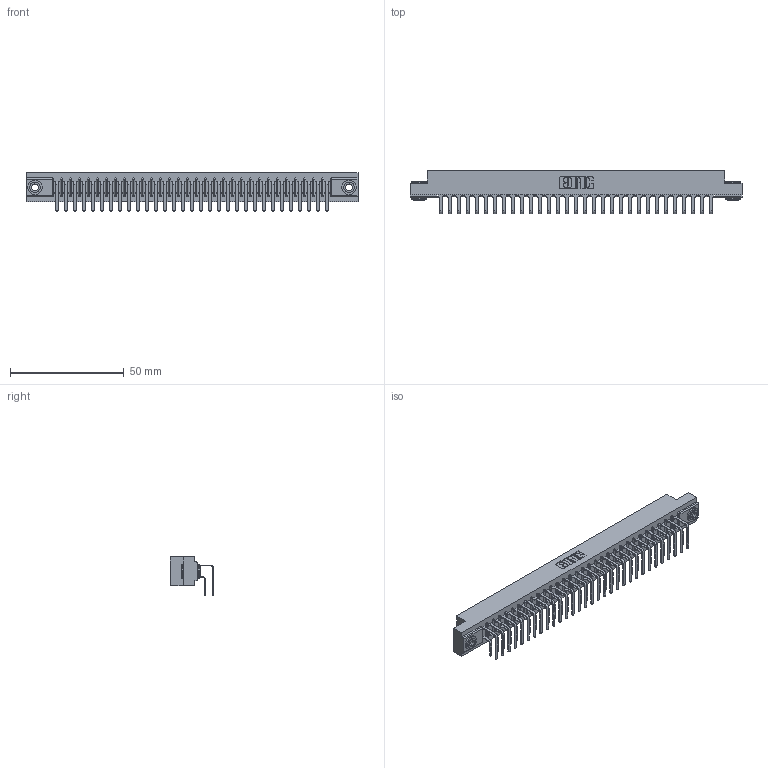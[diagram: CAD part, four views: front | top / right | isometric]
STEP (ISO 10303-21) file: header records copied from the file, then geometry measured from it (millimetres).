
FILE_DESCRIPTION (( 'STEP AP203' ), '1' );
FILE_NAME ('307-062-458-203.STEP', '2020-09-30T16:51:52', ( '' ), ( '' ), 'SwSTEP 2.0', 'SolidWorks 2020', '' );
FILE_SCHEMA (( 'CONFIG_CONTROL_DESIGN' ));
Length unit declared in the file: inch
Products named in the file (5): 307-062-458-203; 307-290-001_558 559 - 1 (Single); 345-250-002_345-250-002-102; 307 Part_.156 Dia Mounting Holes; 307-290-001_558 - 2 (Single)
Assembly tree (65 placements, depth 2):
  307-062-458-203
    307 Part_.156 Dia Mounting Holes
    307-290-001_558 559 - 1 (Single)  x31
    307-290-001_558 - 2 (Single)  x31
    345-250-002_345-250-002-102  x2
Bounding box: 145.85 x 18.96 x 16.8 mm (x, y, z)
Volume: 15707.3 mm3; surface area: 20848.5 mm2
Topology: 65 solids, 65 shells, 3302 faces, 9239 edges, 5986 vertices
Faces by surface type: plane 2140, cylinder 1090, sphere 64, cone 8
Entity records: 31436 total; most frequent: CARTESIAN_POINT 5130, ORIENTED_EDGE 5074, DIRECTION 5043, EDGE_CURVE 2537, VECTOR 1933, LINE 1933, VERTEX_POINT 1642, AXIS2_PLACEMENT_3D 1555
